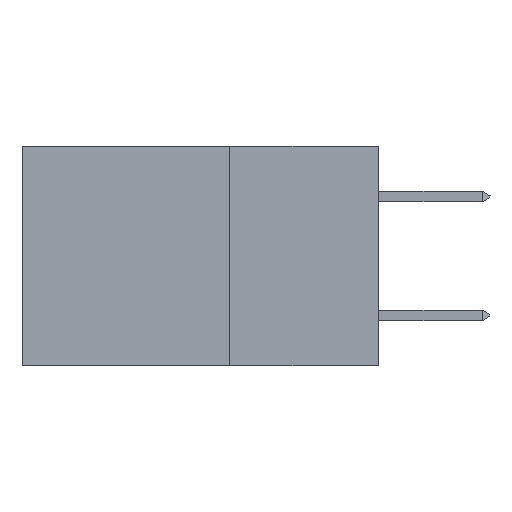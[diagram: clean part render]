
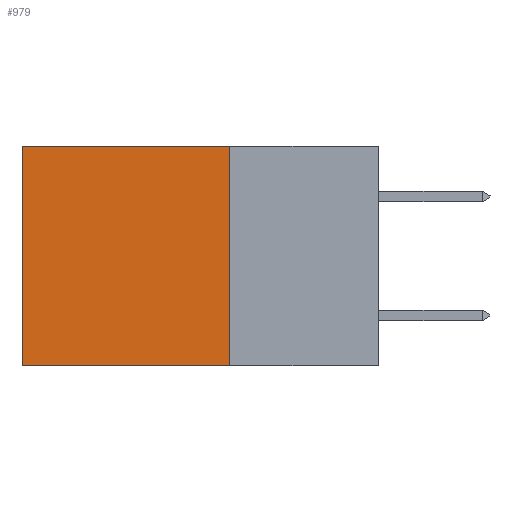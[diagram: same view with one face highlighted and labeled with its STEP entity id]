
A CAD part, left-side view. The second image highlights one B-rep face of the part: STEP entity #979.
In plain terms, the highlighted planar face has unit normal (-1, 0, 0).
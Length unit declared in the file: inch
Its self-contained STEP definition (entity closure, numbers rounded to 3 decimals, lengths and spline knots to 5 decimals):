
#259 = DIRECTION ( 'NONE',  ( 0., 0., -1. ) ) ;
#821 = CARTESIAN_POINT ( 'NONE',  ( 0.2615, 0.6, 0. ) ) ;
#979 = ADVANCED_FACE ( 'NONE', ( #6975 ), #5461, .F. ) ;
#1269 = DIRECTION ( 'NONE',  ( 0., 1., 0. ) ) ;
#1286 = VECTOR ( 'NONE', #8840, 39.37008 ) ;
#1289 = LINE ( 'NONE', #7959, #1286 ) ;
#1847 = ORIENTED_EDGE ( 'NONE', *, *, #8911, .T. ) ;
#3449 = CARTESIAN_POINT ( 'NONE',  ( 0.2615, 0.25, -0.37 ) ) ;
#3483 = LINE ( 'NONE', #5839, #5249 ) ;
#3754 = LINE ( 'NONE', #8883, #6577 ) ;
#3775 = VERTEX_POINT ( 'NONE', #4181 ) ;
#4181 = CARTESIAN_POINT ( 'NONE',  ( 0.2615, 0.25, -0.37 ) ) ;
#4212 = LINE ( 'NONE', #3449, #9926 ) ;
#4280 = EDGE_CURVE ( 'NONE', #3775, #6047, #4212, .T. ) ;
#4928 = EDGE_LOOP ( 'NONE', ( #10121, #10694, #9619, #1847 ) ) ;
#4974 = DIRECTION ( 'NONE',  ( 0., 1., 0. ) ) ;
#5249 = VECTOR ( 'NONE', #6838, 39.37008 ) ;
#5461 = PLANE ( 'NONE',  #8644 ) ;
#5572 = EDGE_CURVE ( 'NONE', #8030, #6047, #3483, .T. ) ;
#5839 = CARTESIAN_POINT ( 'NONE',  ( 0.2615, 0.6, -0.37 ) ) ;
#6047 = VERTEX_POINT ( 'NONE', #7860 ) ;
#6357 = CARTESIAN_POINT ( 'NONE',  ( 0.2615, 0.25, -0.37 ) ) ;
#6577 = VECTOR ( 'NONE', #1269, 39.37008 ) ;
#6817 = CARTESIAN_POINT ( 'NONE',  ( 0.2615, 0.25, 0. ) ) ;
#6838 = DIRECTION ( 'NONE',  ( 0., 0., -1. ) ) ;
#6975 = FACE_OUTER_BOUND ( 'NONE', #4928, .T. ) ;
#7860 = CARTESIAN_POINT ( 'NONE',  ( 0.2615, 0.6, -0.37 ) ) ;
#7959 = CARTESIAN_POINT ( 'NONE',  ( 0.2615, 0.25, -0.37 ) ) ;
#8030 = VERTEX_POINT ( 'NONE', #821 ) ;
#8325 = EDGE_CURVE ( 'NONE', #10222, #3775, #1289, .T. ) ;
#8644 = AXIS2_PLACEMENT_3D ( 'NONE', #6357, #8687, #259 ) ;
#8687 = DIRECTION ( 'NONE',  ( 1., 0., 0. ) ) ;
#8840 = DIRECTION ( 'NONE',  ( 0., 0., -1. ) ) ;
#8883 = CARTESIAN_POINT ( 'NONE',  ( 0.2615, 0.25, 0. ) ) ;
#8911 = EDGE_CURVE ( 'NONE', #10222, #8030, #3754, .T. ) ;
#9619 = ORIENTED_EDGE ( 'NONE', *, *, #8325, .F. ) ;
#9926 = VECTOR ( 'NONE', #4974, 39.37008 ) ;
#10121 = ORIENTED_EDGE ( 'NONE', *, *, #5572, .T. ) ;
#10222 = VERTEX_POINT ( 'NONE', #6817 ) ;
#10694 = ORIENTED_EDGE ( 'NONE', *, *, #4280, .F. ) ;
